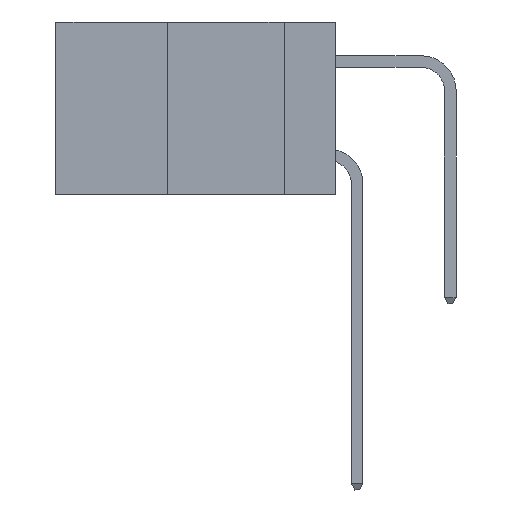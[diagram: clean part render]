
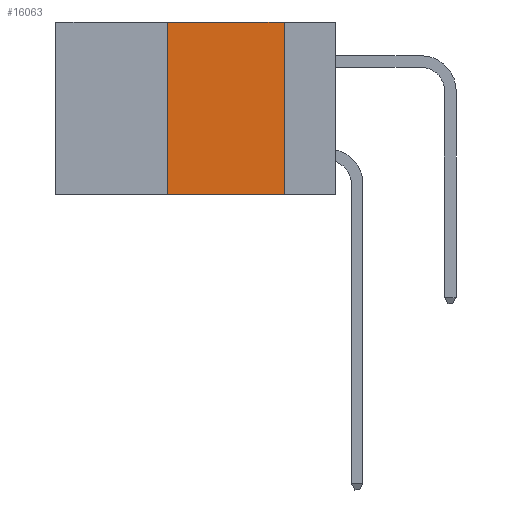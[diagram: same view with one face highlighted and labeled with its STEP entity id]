
A CAD part, left-side view. The second image highlights one B-rep face of the part: STEP entity #16063.
In plain terms, the highlighted planar face has unit normal (-1, 0, 0).
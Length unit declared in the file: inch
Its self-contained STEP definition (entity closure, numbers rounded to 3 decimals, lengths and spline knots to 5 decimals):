
#310 = CARTESIAN_POINT ( 'NONE',  ( 0., 0.6, -0.37 ) ) ;
#375 = DIRECTION ( 'NONE',  ( 0., -1., 0. ) ) ;
#748 = EDGE_LOOP ( 'NONE', ( #6772, #11220, #7725, #15846 ) ) ;
#951 = CARTESIAN_POINT ( 'NONE',  ( 0., 0.36, 0. ) ) ;
#1186 = CARTESIAN_POINT ( 'NONE',  ( 0., 0.11, 0. ) ) ;
#1638 = VECTOR ( 'NONE', #14981, 39.37008 ) ;
#1740 = VERTEX_POINT ( 'NONE', #1186 ) ;
#1826 = PLANE ( 'NONE',  #9234 ) ;
#3150 = VECTOR ( 'NONE', #17261, 39.37008 ) ;
#3236 = CARTESIAN_POINT ( 'NONE',  ( 0., 0.11, 0. ) ) ;
#3437 = DIRECTION ( 'NONE',  ( 1., 0., 0. ) ) ;
#3509 = VECTOR ( 'NONE', #375, 39.37008 ) ;
#4246 = EDGE_CURVE ( 'NONE', #1740, #10896, #16842, .T. ) ;
#5698 = CARTESIAN_POINT ( 'NONE',  ( 0., 0.6, 0. ) ) ;
#6772 = ORIENTED_EDGE ( 'NONE', *, *, #4246, .F. ) ;
#7215 = LINE ( 'NONE', #5698, #3150 ) ;
#7725 = ORIENTED_EDGE ( 'NONE', *, *, #16933, .F. ) ;
#8659 = CARTESIAN_POINT ( 'NONE',  ( 0., 0.11, -0.37 ) ) ;
#9234 = AXIS2_PLACEMENT_3D ( 'NONE', #12390, #3437, #13818 ) ;
#10463 = DIRECTION ( 'NONE',  ( 0., 0., 1. ) ) ;
#10752 = VECTOR ( 'NONE', #10463, 39.37008 ) ;
#10896 = VERTEX_POINT ( 'NONE', #8659 ) ;
#11220 = ORIENTED_EDGE ( 'NONE', *, *, #17420, .F. ) ;
#12390 = CARTESIAN_POINT ( 'NONE',  ( 0., 0.6, 0. ) ) ;
#13445 = FACE_OUTER_BOUND ( 'NONE', #748, .T. ) ;
#13818 = DIRECTION ( 'NONE',  ( 0., 0., -1. ) ) ;
#14981 = DIRECTION ( 'NONE',  ( 0., 0., -1. ) ) ;
#15638 = CARTESIAN_POINT ( 'NONE',  ( 0., 0.36, -0.37 ) ) ;
#15846 = ORIENTED_EDGE ( 'NONE', *, *, #18471, .T. ) ;
#16063 = ADVANCED_FACE ( 'NONE', ( #13445 ), #1826, .F. ) ;
#16146 = LINE ( 'NONE', #310, #3509 ) ;
#16207 = VERTEX_POINT ( 'NONE', #951 ) ;
#16842 = LINE ( 'NONE', #3236, #1638 ) ;
#16933 = EDGE_CURVE ( 'NONE', #18562, #16207, #18224, .T. ) ;
#17261 = DIRECTION ( 'NONE',  ( 0., -1., 0. ) ) ;
#17420 = EDGE_CURVE ( 'NONE', #16207, #1740, #7215, .T. ) ;
#17462 = CARTESIAN_POINT ( 'NONE',  ( 0., 0.36, 0. ) ) ;
#18224 = LINE ( 'NONE', #17462, #10752 ) ;
#18471 = EDGE_CURVE ( 'NONE', #18562, #10896, #16146, .T. ) ;
#18562 = VERTEX_POINT ( 'NONE', #15638 ) ;
